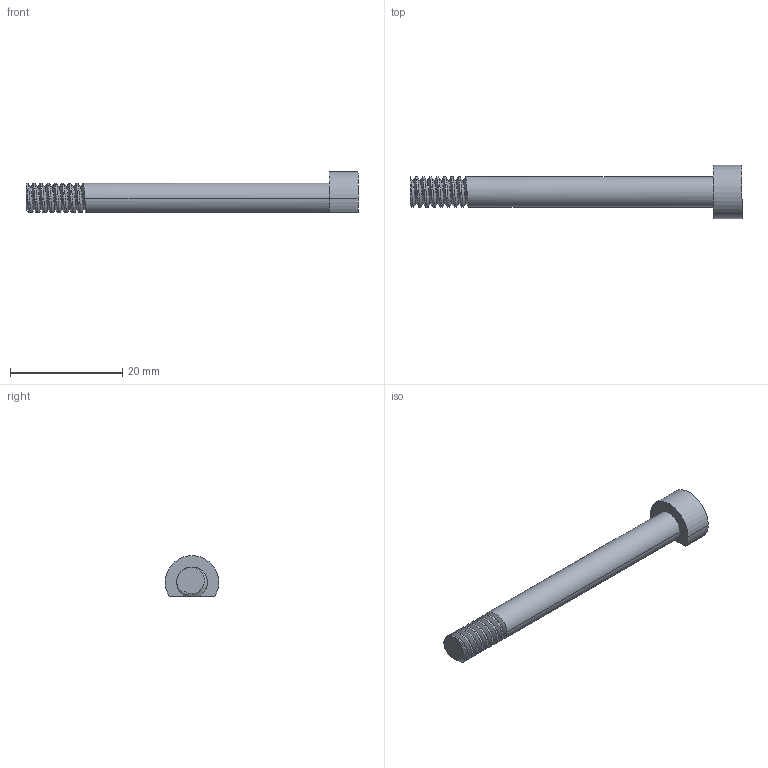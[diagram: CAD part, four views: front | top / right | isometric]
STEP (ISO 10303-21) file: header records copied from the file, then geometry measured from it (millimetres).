
FILE_DESCRIPTION (( 'STEP AP203' ), '1' );
FILE_NAME ('AF-WF-VF-PRT-002-STEP.STEP', '2020-07-22T01:01:52', ( '' ), ( '' ), 'SwSTEP 2.0', 'SolidWorks 2018', '' );
FILE_SCHEMA (( 'CONFIG_CONTROL_DESIGN' ));
Length unit declared in the file: inch
Products named in the file (1): AF-WF-VF-PRT-002-STEP
Bounding box: 59.05 x 9.53 x 7.24 mm (x, y, z)
Volume: 1472.8 mm3; surface area: 1294.1 mm2
Topology: 1 solids, 1 shells, 52 faces, 148 edges, 98 vertices
Faces by surface type: cylinder 33, plane 16, bspline 3
Entity records: 3071 total; most frequent: CARTESIAN_POINT 1830, ORIENTED_EDGE 296, DIRECTION 191, EDGE_CURVE 148, VERTEX_POINT 98, AXIS2_PLACEMENT_3D 66, VECTOR 59, LINE 59
